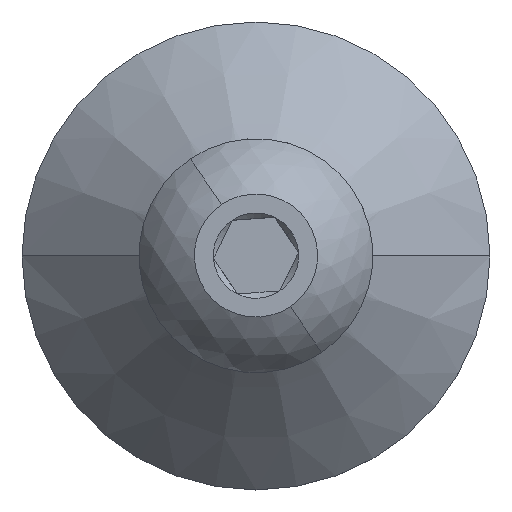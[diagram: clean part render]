
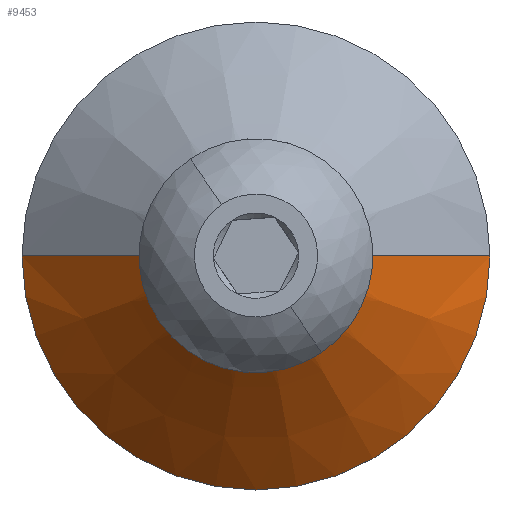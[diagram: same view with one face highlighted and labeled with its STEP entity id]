
A CAD part, top view. The second image highlights one B-rep face of the part: STEP entity #9453.
In plain terms, the highlighted conical face has half-angle 45 degrees and reference radius 9.5 mm.
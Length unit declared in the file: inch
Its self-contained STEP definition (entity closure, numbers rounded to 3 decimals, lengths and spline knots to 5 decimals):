
#397 = LINE ( 'NONE', #18295, #20362 ) ;
#2056 = CARTESIAN_POINT ( 'NONE',  ( -0.13279, 0., -0.00879 ) ) ;
#2378 = EDGE_CURVE ( 'NONE', #4357, #9538, #6315, .T. ) ;
#2404 = DIRECTION ( 'NONE',  ( 0., 0., -1. ) ) ;
#3112 = DIRECTION ( 'NONE',  ( -0.707, 0., -0.707 ) ) ;
#3302 = ORIENTED_EDGE ( 'NONE', *, *, #9367, .T. ) ;
#3810 = EDGE_LOOP ( 'NONE', ( #5364, #16566, #3302, #11772 ) ) ;
#3908 = CARTESIAN_POINT ( 'NONE',  ( 0., 0., -0.00879 ) ) ;
#4357 = VERTEX_POINT ( 'NONE', #12420 ) ;
#4544 = AXIS2_PLACEMENT_3D ( 'NONE', #12923, #19501, #4727 ) ;
#4727 = DIRECTION ( 'NONE',  ( -1., 0., 0. ) ) ;
#4892 = DIRECTION ( 'NONE',  ( 0., 0., 1. ) ) ;
#5364 = ORIENTED_EDGE ( 'NONE', *, *, #18249, .F. ) ;
#5945 = DIRECTION ( 'NONE',  ( 1., 0., 0. ) ) ;
#6315 = CIRCLE ( 'NONE', #14585, 0.13279 ) ;
#6955 = DIRECTION ( 'NONE',  ( 0.707, 0., -0.707 ) ) ;
#8009 = EDGE_CURVE ( 'NONE', #12663, #14125, #11428, .T. ) ;
#8344 = CONICAL_SURFACE ( 'NONE', #4544, 0.374, 0.785 ) ;
#8447 = CARTESIAN_POINT ( 'NONE',  ( -0.374, 0., -0.25 ) ) ;
#8457 = DIRECTION ( 'NONE',  ( 1., 0., 0. ) ) ;
#9367 = EDGE_CURVE ( 'NONE', #9538, #12663, #10017, .T. ) ;
#9453 = ADVANCED_FACE ( 'NONE', ( #17789 ), #8344, .T. ) ;
#9538 = VERTEX_POINT ( 'NONE', #2056 ) ;
#10017 = LINE ( 'NONE', #14539, #12798 ) ;
#11428 = CIRCLE ( 'NONE', #19688, 0.374 ) ;
#11772 = ORIENTED_EDGE ( 'NONE', *, *, #8009, .T. ) ;
#12420 = CARTESIAN_POINT ( 'NONE',  ( 0.13279, 0., -0.00879 ) ) ;
#12663 = VERTEX_POINT ( 'NONE', #8447 ) ;
#12798 = VECTOR ( 'NONE', #3112, 39.37008 ) ;
#12923 = CARTESIAN_POINT ( 'NONE',  ( 0., 0., -0.25 ) ) ;
#14125 = VERTEX_POINT ( 'NONE', #16084 ) ;
#14539 = CARTESIAN_POINT ( 'NONE',  ( -0.374, 0., -0.25 ) ) ;
#14585 = AXIS2_PLACEMENT_3D ( 'NONE', #3908, #2404, #5945 ) ;
#16084 = CARTESIAN_POINT ( 'NONE',  ( 0.374, 0., -0.25 ) ) ;
#16566 = ORIENTED_EDGE ( 'NONE', *, *, #2378, .T. ) ;
#17789 = FACE_OUTER_BOUND ( 'NONE', #3810, .T. ) ;
#18249 = EDGE_CURVE ( 'NONE', #4357, #14125, #397, .T. ) ;
#18295 = CARTESIAN_POINT ( 'NONE',  ( 0.374, 0., -0.25 ) ) ;
#19501 = DIRECTION ( 'NONE',  ( 0., 0., -1. ) ) ;
#19688 = AXIS2_PLACEMENT_3D ( 'NONE', #21173, #4892, #8457 ) ;
#20362 = VECTOR ( 'NONE', #6955, 39.37008 ) ;
#21173 = CARTESIAN_POINT ( 'NONE',  ( 0., 0., -0.25 ) ) ;
